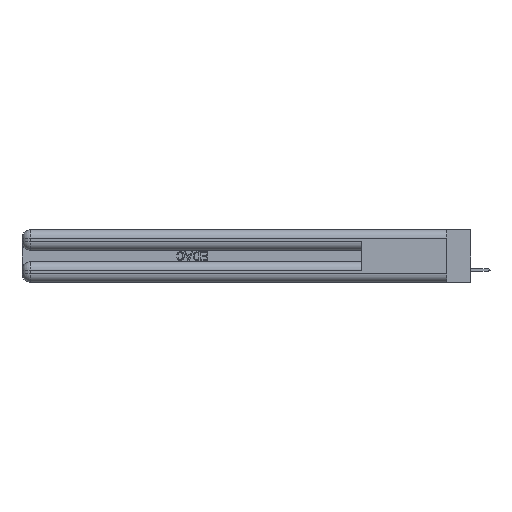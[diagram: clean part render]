
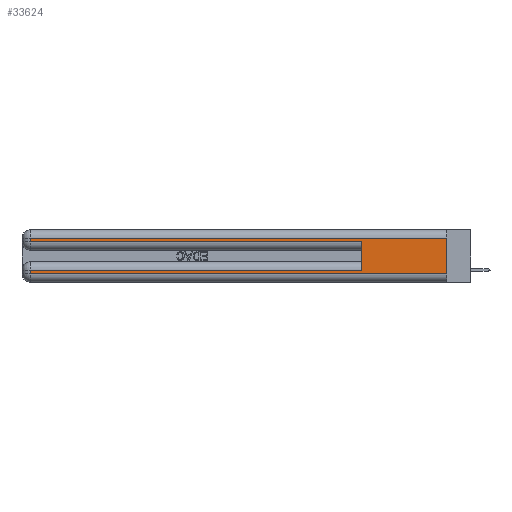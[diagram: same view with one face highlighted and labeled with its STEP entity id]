
A CAD part, left-side view. The second image highlights one B-rep face of the part: STEP entity #33624.
In plain terms, the highlighted planar face has unit normal (-1, 0, 0).
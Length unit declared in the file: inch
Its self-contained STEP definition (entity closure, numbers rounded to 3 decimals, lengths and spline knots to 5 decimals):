
#497 = VECTOR ( 'NONE', #30835, 39.37008 ) ;
#968 = VERTEX_POINT ( 'NONE', #43331 ) ;
#2406 = VECTOR ( 'NONE', #42998, 39.37008 ) ;
#2428 = CARTESIAN_POINT ( 'NONE',  ( 0., 2.94, 0.37 ) ) ;
#2726 = ORIENTED_EDGE ( 'NONE', *, *, #10973, .T. ) ;
#4089 = LINE ( 'NONE', #24279, #25209 ) ;
#4319 = CARTESIAN_POINT ( 'NONE',  ( 0., 0.6, 0.285 ) ) ;
#4489 = CARTESIAN_POINT ( 'NONE',  ( 0., 0., 0.37 ) ) ;
#5515 = DIRECTION ( 'NONE',  ( 0., 0., -1. ) ) ;
#6074 = EDGE_CURVE ( 'NONE', #968, #17229, #46625, .T. ) ;
#6315 = CARTESIAN_POINT ( 'NONE',  ( 0., 2.94, 0.285 ) ) ;
#7757 = DIRECTION ( 'NONE',  ( 0., 1., 0. ) ) ;
#8662 = VERTEX_POINT ( 'NONE', #6315 ) ;
#9359 = ORIENTED_EDGE ( 'NONE', *, *, #37738, .T. ) ;
#10031 = LINE ( 'NONE', #2428, #18472 ) ;
#10973 = EDGE_CURVE ( 'NONE', #13869, #22232, #26636, .T. ) ;
#11256 = EDGE_CURVE ( 'NONE', #44648, #25240, #34196, .T. ) ;
#13376 = EDGE_CURVE ( 'NONE', #22232, #17229, #18410, .T. ) ;
#13869 = VERTEX_POINT ( 'NONE', #31928 ) ;
#14210 = CARTESIAN_POINT ( 'NONE',  ( 0., 0., 0.06 ) ) ;
#16385 = DIRECTION ( 'NONE',  ( 0., 1., 0. ) ) ;
#17229 = VERTEX_POINT ( 'NONE', #51584 ) ;
#17305 = FACE_OUTER_BOUND ( 'NONE', #19108, .T. ) ;
#17963 = EDGE_CURVE ( 'NONE', #8662, #25240, #51135, .T. ) ;
#18410 = LINE ( 'NONE', #14210, #49122 ) ;
#18472 = VECTOR ( 'NONE', #34422, 39.37008 ) ;
#18868 = CARTESIAN_POINT ( 'NONE',  ( 0., 0., 0.285 ) ) ;
#19108 = EDGE_LOOP ( 'NONE', ( #44992, #45630, #40958, #36124, #46915, #9359, #2726, #31883 ) ) ;
#19262 = EDGE_CURVE ( 'NONE', #36121, #8662, #10031, .T. ) ;
#20658 = CARTESIAN_POINT ( 'NONE',  ( 0., 2.94, 0.31 ) ) ;
#22232 = VERTEX_POINT ( 'NONE', #44946 ) ;
#24279 = CARTESIAN_POINT ( 'NONE',  ( 0., 0., 0.31 ) ) ;
#24440 = VECTOR ( 'NONE', #26667, 39.37008 ) ;
#25209 = VECTOR ( 'NONE', #16385, 39.37008 ) ;
#25240 = VERTEX_POINT ( 'NONE', #4319 ) ;
#25816 = DIRECTION ( 'NONE',  ( 0., 0., 1. ) ) ;
#26636 = LINE ( 'NONE', #47624, #497 ) ;
#26667 = DIRECTION ( 'NONE',  ( 0., 0., -1. ) ) ;
#27962 = CARTESIAN_POINT ( 'NONE',  ( 0., 0., 0.085 ) ) ;
#29542 = AXIS2_PLACEMENT_3D ( 'NONE', #4489, #49327, #5515 ) ;
#30835 = DIRECTION ( 'NONE',  ( 0., 0., -1. ) ) ;
#31883 = ORIENTED_EDGE ( 'NONE', *, *, #13376, .T. ) ;
#31928 = CARTESIAN_POINT ( 'NONE',  ( 0., 2.94, 0.085 ) ) ;
#33471 = VECTOR ( 'NONE', #7757, 39.37008 ) ;
#33624 = ADVANCED_FACE ( 'NONE', ( #17305 ), #36729, .F. ) ;
#34196 = LINE ( 'NONE', #37877, #51463 ) ;
#34422 = DIRECTION ( 'NONE',  ( 0., 0., -1. ) ) ;
#35194 = DIRECTION ( 'NONE',  ( 0., -1., 0. ) ) ;
#36121 = VERTEX_POINT ( 'NONE', #20658 ) ;
#36124 = ORIENTED_EDGE ( 'NONE', *, *, #17963, .T. ) ;
#36729 = PLANE ( 'NONE',  #29542 ) ;
#37636 = EDGE_CURVE ( 'NONE', #968, #36121, #4089, .T. ) ;
#37738 = EDGE_CURVE ( 'NONE', #44648, #13869, #43691, .T. ) ;
#37877 = CARTESIAN_POINT ( 'NONE',  ( 0., 0.6, 0.145 ) ) ;
#40958 = ORIENTED_EDGE ( 'NONE', *, *, #19262, .T. ) ;
#42998 = DIRECTION ( 'NONE',  ( 0., -1., 0. ) ) ;
#43331 = CARTESIAN_POINT ( 'NONE',  ( 0., 0., 0.31 ) ) ;
#43691 = LINE ( 'NONE', #27962, #33471 ) ;
#44648 = VERTEX_POINT ( 'NONE', #44686 ) ;
#44686 = CARTESIAN_POINT ( 'NONE',  ( 0., 0.6, 0.085 ) ) ;
#44946 = CARTESIAN_POINT ( 'NONE',  ( 0., 2.94, 0.06 ) ) ;
#44992 = ORIENTED_EDGE ( 'NONE', *, *, #6074, .F. ) ;
#45630 = ORIENTED_EDGE ( 'NONE', *, *, #37636, .T. ) ;
#46625 = LINE ( 'NONE', #50299, #24440 ) ;
#46915 = ORIENTED_EDGE ( 'NONE', *, *, #11256, .F. ) ;
#47624 = CARTESIAN_POINT ( 'NONE',  ( 0., 2.94, 0.37 ) ) ;
#49122 = VECTOR ( 'NONE', #35194, 39.37008 ) ;
#49327 = DIRECTION ( 'NONE',  ( 1., 0., 0. ) ) ;
#50299 = CARTESIAN_POINT ( 'NONE',  ( 0., 0., 0.37 ) ) ;
#51135 = LINE ( 'NONE', #18868, #2406 ) ;
#51463 = VECTOR ( 'NONE', #25816, 39.37008 ) ;
#51584 = CARTESIAN_POINT ( 'NONE',  ( 0., 0., 0.06 ) ) ;
